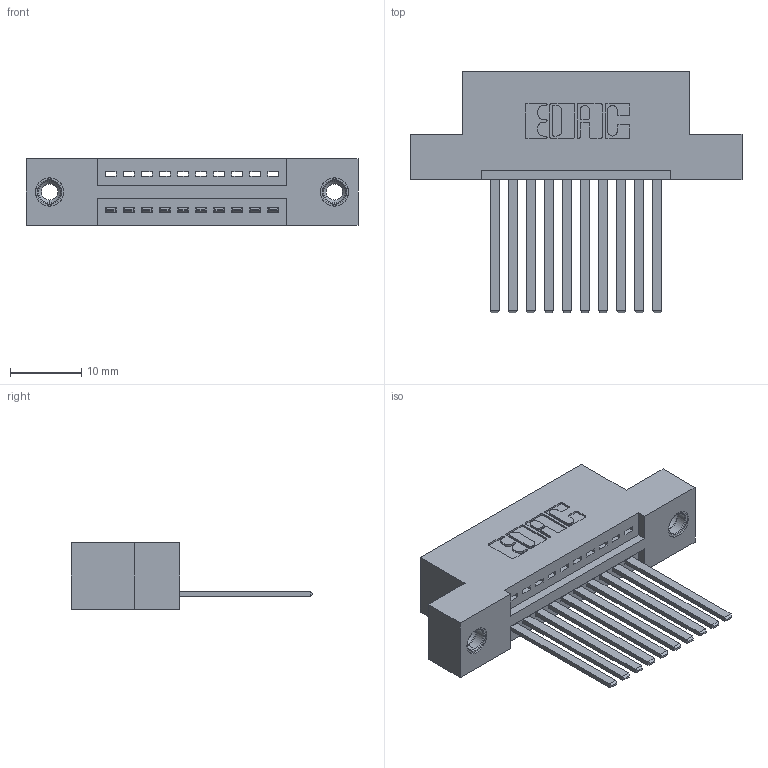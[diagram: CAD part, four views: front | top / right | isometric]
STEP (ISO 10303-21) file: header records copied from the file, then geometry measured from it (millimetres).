
FILE_DESCRIPTION (( 'STEP AP203' ), '1' );
FILE_NAME ('395-010-544-108.STEP', '2018-10-24T06:35:29', ( '' ), ( '' ), 'SwSTEP 2.0', 'SolidWorks 2016', '' );
FILE_SCHEMA (( 'CONFIG_CONTROL_DESIGN' ));
Length unit declared in the file: inch
Products named in the file (4): 395-010-544-108; 345-250-001_345-250-003-102; 345-292-001_345-293-144; 345 Part_Flush Mounting Lugs - 0.156 Dia-TI
Assembly tree (13 placements, depth 2):
  395-010-544-108
    345 Part_Flush Mounting Lugs - 0.156 Dia-TI
    345-292-001_345-293-144  x10
    345-250-001_345-250-003-102  x2
Bounding box: 46.61 x 33.96 x 9.4 mm (x, y, z)
Volume: 4274.1 mm3; surface area: 5611.9 mm2
Topology: 13 solids, 13 shells, 706 faces, 2057 edges, 1350 vertices
Faces by surface type: plane 472, cylinder 218, cone 12, torus 4
Entity records: 12836 total; most frequent: CARTESIAN_POINT 2205, ORIENTED_EDGE 2142, DIRECTION 1997, EDGE_CURVE 1071, LINE 883, VECTOR 883, VERTEX_POINT 708, AXIS2_PLACEMENT_3D 557
